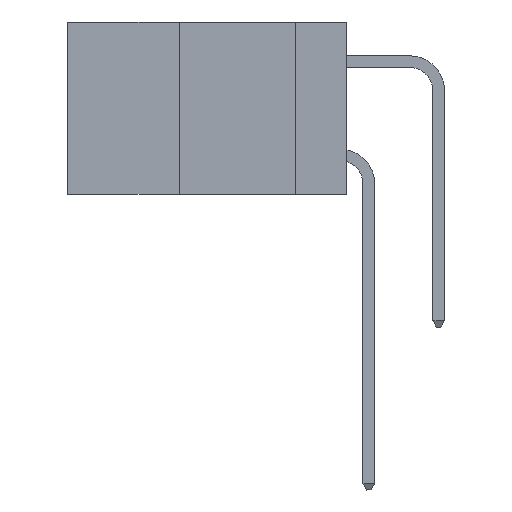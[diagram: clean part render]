
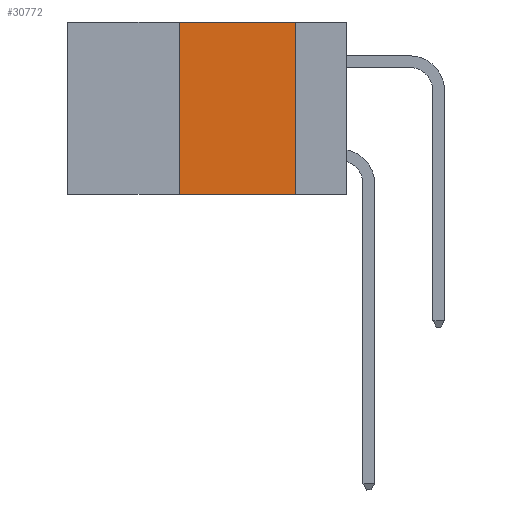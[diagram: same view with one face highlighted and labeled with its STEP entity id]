
A CAD part, left-side view. The second image highlights one B-rep face of the part: STEP entity #30772.
In plain terms, the highlighted planar face has unit normal (-1, 0, 0).
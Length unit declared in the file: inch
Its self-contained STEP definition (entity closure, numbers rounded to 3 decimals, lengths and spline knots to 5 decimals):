
#502 = VERTEX_POINT ( 'NONE', #26293 ) ;
#856 = VECTOR ( 'NONE', #11638, 39.37008 ) ;
#2157 = DIRECTION ( 'NONE',  ( 0., -1., 0. ) ) ;
#2727 = PLANE ( 'NONE',  #7046 ) ;
#4304 = VECTOR ( 'NONE', #2157, 39.37008 ) ;
#6045 = CARTESIAN_POINT ( 'NONE',  ( 0., 0.11, 0. ) ) ;
#7046 = AXIS2_PLACEMENT_3D ( 'NONE', #21626, #14624, #35399 ) ;
#7958 = LINE ( 'NONE', #23957, #27051 ) ;
#8046 = ORIENTED_EDGE ( 'NONE', *, *, #35708, .F. ) ;
#8742 = VERTEX_POINT ( 'NONE', #26130 ) ;
#8954 = EDGE_CURVE ( 'NONE', #8742, #13979, #7958, .T. ) ;
#9376 = LINE ( 'NONE', #29184, #15078 ) ;
#10480 = CARTESIAN_POINT ( 'NONE',  ( 0., 0.36, -0.37 ) ) ;
#10531 = FACE_OUTER_BOUND ( 'NONE', #10847, .T. ) ;
#10847 = EDGE_LOOP ( 'NONE', ( #8046, #22610, #25279, #17111 ) ) ;
#11638 = DIRECTION ( 'NONE',  ( 0., 0., -1. ) ) ;
#13979 = VERTEX_POINT ( 'NONE', #31421 ) ;
#14624 = DIRECTION ( 'NONE',  ( 1., 0., 0. ) ) ;
#15078 = VECTOR ( 'NONE', #25759, 39.37008 ) ;
#17111 = ORIENTED_EDGE ( 'NONE', *, *, #33228, .T. ) ;
#21626 = CARTESIAN_POINT ( 'NONE',  ( 0., 0.6, 0. ) ) ;
#22610 = ORIENTED_EDGE ( 'NONE', *, *, #8954, .F. ) ;
#23957 = CARTESIAN_POINT ( 'NONE',  ( 0., 0.6, 0. ) ) ;
#24162 = CARTESIAN_POINT ( 'NONE',  ( 0., 0.6, -0.37 ) ) ;
#24509 = DIRECTION ( 'NONE',  ( 0., -1., 0. ) ) ;
#25279 = ORIENTED_EDGE ( 'NONE', *, *, #29092, .F. ) ;
#25577 = VERTEX_POINT ( 'NONE', #10480 ) ;
#25759 = DIRECTION ( 'NONE',  ( 0., 0., 1. ) ) ;
#26130 = CARTESIAN_POINT ( 'NONE',  ( 0., 0.36, 0. ) ) ;
#26293 = CARTESIAN_POINT ( 'NONE',  ( 0., 0.11, -0.37 ) ) ;
#27051 = VECTOR ( 'NONE', #24509, 39.37008 ) ;
#29092 = EDGE_CURVE ( 'NONE', #25577, #8742, #9376, .T. ) ;
#29184 = CARTESIAN_POINT ( 'NONE',  ( 0., 0.36, 0. ) ) ;
#30772 = ADVANCED_FACE ( 'NONE', ( #10531 ), #2727, .F. ) ;
#31421 = CARTESIAN_POINT ( 'NONE',  ( 0., 0.11, 0. ) ) ;
#31918 = LINE ( 'NONE', #24162, #4304 ) ;
#33228 = EDGE_CURVE ( 'NONE', #25577, #502, #31918, .T. ) ;
#34506 = LINE ( 'NONE', #6045, #856 ) ;
#35399 = DIRECTION ( 'NONE',  ( 0., 0., -1. ) ) ;
#35708 = EDGE_CURVE ( 'NONE', #13979, #502, #34506, .T. ) ;
